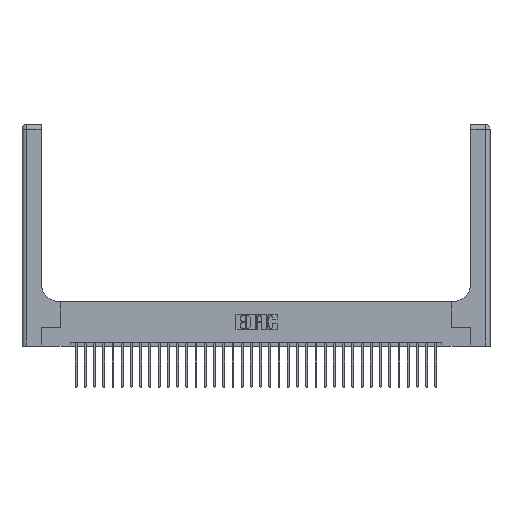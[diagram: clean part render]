
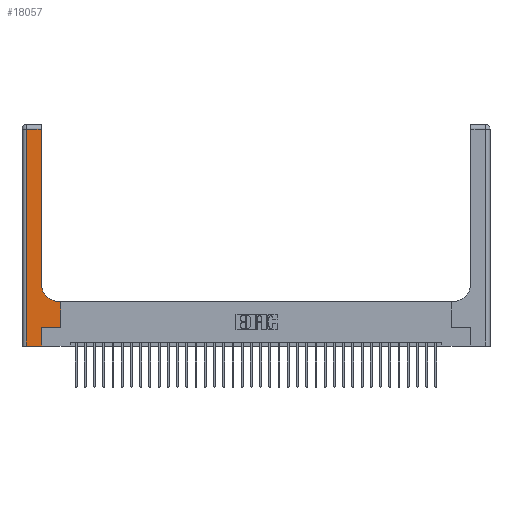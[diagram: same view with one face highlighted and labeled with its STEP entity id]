
A CAD part, top view. The second image highlights one B-rep face of the part: STEP entity #18057.
In plain terms, the highlighted planar face has unit normal (0, 0, 1).
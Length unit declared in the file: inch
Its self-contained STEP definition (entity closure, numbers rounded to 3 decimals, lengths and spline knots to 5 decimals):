
#149 = VERTEX_POINT ( 'NONE', #17456 ) ;
#150 = EDGE_CURVE ( 'NONE', #4052, #6835, #15646, .T. ) ;
#492 = ORIENTED_EDGE ( 'NONE', *, *, #11359, .T. ) ;
#559 = CARTESIAN_POINT ( 'NONE',  ( 0.265, 0.25, 0.37 ) ) ;
#939 = CARTESIAN_POINT ( 'NONE',  ( 0.26, 3., 0.37 ) ) ;
#1015 = EDGE_CURVE ( 'NONE', #17273, #13396, #15377, .T. ) ;
#1909 = EDGE_CURVE ( 'NONE', #149, #22893, #9950, .T. ) ;
#2241 = ORIENTED_EDGE ( 'NONE', *, *, #22633, .T. ) ;
#2421 = DIRECTION ( 'NONE',  ( 0., 1., 0. ) ) ;
#2690 = CARTESIAN_POINT ( 'NONE',  ( 0.528, 0.6, 0.37 ) ) ;
#3601 = VECTOR ( 'NONE', #6525, 39.37008 ) ;
#4005 = CARTESIAN_POINT ( 'NONE',  ( 0., 0., 0.37 ) ) ;
#4052 = VERTEX_POINT ( 'NONE', #20301 ) ;
#4074 = CARTESIAN_POINT ( 'NONE',  ( 0., 3., 0.37 ) ) ;
#5266 = VERTEX_POINT ( 'NONE', #27171 ) ;
#5427 = DIRECTION ( 'NONE',  ( 1., 0., 0. ) ) ;
#5994 = ORIENTED_EDGE ( 'NONE', *, *, #1909, .T. ) ;
#6351 = LINE ( 'NONE', #13830, #3601 ) ;
#6525 = DIRECTION ( 'NONE',  ( 0., 1., 0. ) ) ;
#6835 = VERTEX_POINT ( 'NONE', #24921 ) ;
#7155 = ORIENTED_EDGE ( 'NONE', *, *, #150, .T. ) ;
#7403 = DIRECTION ( 'NONE',  ( -1., 0., 0. ) ) ;
#9347 = CIRCLE ( 'NONE', #21764, 0.25 ) ;
#9488 = CARTESIAN_POINT ( 'NONE',  ( 0.51, 0.6, 0.37 ) ) ;
#9909 = ORIENTED_EDGE ( 'NONE', *, *, #25300, .T. ) ;
#9950 = LINE ( 'NONE', #16609, #23571 ) ;
#10680 = DIRECTION ( 'NONE',  ( 1., 0., 0. ) ) ;
#10703 = AXIS2_PLACEMENT_3D ( 'NONE', #4074, #21433, #31323 ) ;
#11276 = CARTESIAN_POINT ( 'NONE',  ( 0.06, 0., 0.37 ) ) ;
#11359 = EDGE_CURVE ( 'NONE', #5266, #11529, #28002, .T. ) ;
#11529 = VERTEX_POINT ( 'NONE', #16837 ) ;
#11535 = ORIENTED_EDGE ( 'NONE', *, *, #17048, .T. ) ;
#12440 = CARTESIAN_POINT ( 'NONE',  ( 0., 2.94, 0.37 ) ) ;
#13396 = VERTEX_POINT ( 'NONE', #9488 ) ;
#13830 = CARTESIAN_POINT ( 'NONE',  ( 0.265, 0., 0.37 ) ) ;
#15350 = VECTOR ( 'NONE', #2421, 39.37008 ) ;
#15377 = LINE ( 'NONE', #30267, #31277 ) ;
#15646 = LINE ( 'NONE', #559, #22051 ) ;
#16609 = CARTESIAN_POINT ( 'NONE',  ( 0.06, 3., 0.37 ) ) ;
#16837 = CARTESIAN_POINT ( 'NONE',  ( 0.26, 2.94, 0.37 ) ) ;
#17048 = EDGE_CURVE ( 'NONE', #6835, #17273, #29961, .T. ) ;
#17273 = VERTEX_POINT ( 'NONE', #2690 ) ;
#17456 = CARTESIAN_POINT ( 'NONE',  ( 0.06, 2.94, 0.37 ) ) ;
#18057 = ADVANCED_FACE ( 'NONE', ( #21273 ), #31157, .F. ) ;
#18769 = VECTOR ( 'NONE', #21201, 39.37008 ) ;
#18971 = DIRECTION ( 'NONE',  ( 0., 0., -1. ) ) ;
#20301 = CARTESIAN_POINT ( 'NONE',  ( 0.265, 0.25, 0.37 ) ) ;
#20308 = ORIENTED_EDGE ( 'NONE', *, *, #1015, .T. ) ;
#21201 = DIRECTION ( 'NONE',  ( 0., 1., 0. ) ) ;
#21273 = FACE_OUTER_BOUND ( 'NONE', #23436, .T. ) ;
#21433 = DIRECTION ( 'NONE',  ( 0., 0., -1. ) ) ;
#21764 = AXIS2_PLACEMENT_3D ( 'NONE', #31119, #18971, #28695 ) ;
#21878 = VECTOR ( 'NONE', #10680, 39.37008 ) ;
#22051 = VECTOR ( 'NONE', #5427, 39.37008 ) ;
#22219 = EDGE_CURVE ( 'NONE', #28795, #4052, #6351, .T. ) ;
#22633 = EDGE_CURVE ( 'NONE', #11529, #149, #27645, .T. ) ;
#22893 = VERTEX_POINT ( 'NONE', #11276 ) ;
#23436 = EDGE_LOOP ( 'NONE', ( #492, #2241, #5994, #9909, #30300, #7155, #11535, #20308, #27660 ) ) ;
#23571 = VECTOR ( 'NONE', #26462, 39.37008 ) ;
#24355 = VECTOR ( 'NONE', #7403, 39.37008 ) ;
#24635 = CARTESIAN_POINT ( 'NONE',  ( 0.528, 0.25, 0.37 ) ) ;
#24921 = CARTESIAN_POINT ( 'NONE',  ( 0.528, 0.25, 0.37 ) ) ;
#25300 = EDGE_CURVE ( 'NONE', #22893, #28795, #26210, .T. ) ;
#26210 = LINE ( 'NONE', #4005, #21878 ) ;
#26462 = DIRECTION ( 'NONE',  ( 0., -1., 0. ) ) ;
#27171 = CARTESIAN_POINT ( 'NONE',  ( 0.26, 0.85, 0.37 ) ) ;
#27645 = LINE ( 'NONE', #12440, #24355 ) ;
#27660 = ORIENTED_EDGE ( 'NONE', *, *, #31165, .T. ) ;
#28002 = LINE ( 'NONE', #939, #18769 ) ;
#28695 = DIRECTION ( 'NONE',  ( 1., 0., 0. ) ) ;
#28795 = VERTEX_POINT ( 'NONE', #29755 ) ;
#29755 = CARTESIAN_POINT ( 'NONE',  ( 0.265, 0., 0.37 ) ) ;
#29961 = LINE ( 'NONE', #24635, #15350 ) ;
#30267 = CARTESIAN_POINT ( 'NONE',  ( 0.26, 0.6, 0.37 ) ) ;
#30300 = ORIENTED_EDGE ( 'NONE', *, *, #22219, .T. ) ;
#30421 = DIRECTION ( 'NONE',  ( -1., 0., 0. ) ) ;
#31119 = CARTESIAN_POINT ( 'NONE',  ( 0.51, 0.85, 0.37 ) ) ;
#31157 = PLANE ( 'NONE',  #10703 ) ;
#31165 = EDGE_CURVE ( 'NONE', #13396, #5266, #9347, .T. ) ;
#31277 = VECTOR ( 'NONE', #30421, 39.37008 ) ;
#31323 = DIRECTION ( 'NONE',  ( -1., 0., 0. ) ) ;
